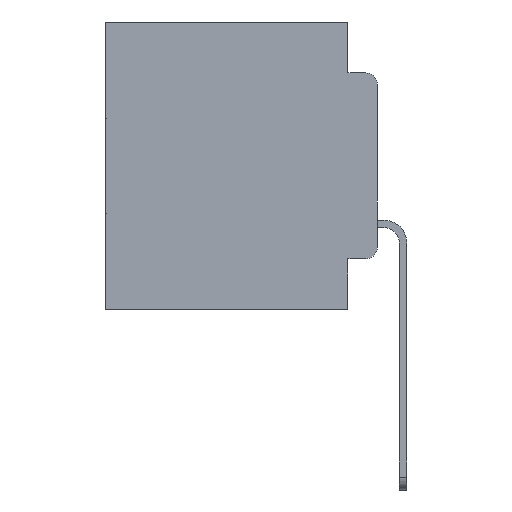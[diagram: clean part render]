
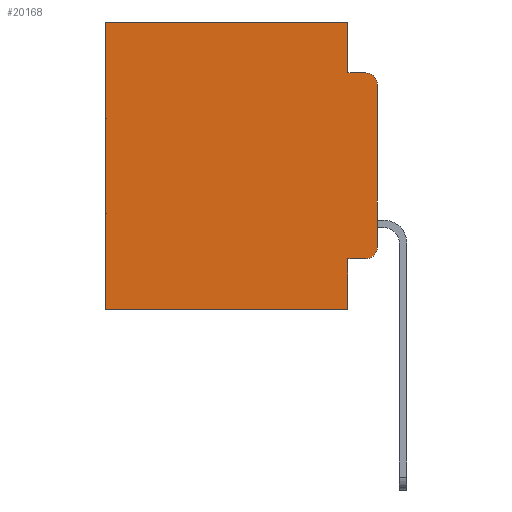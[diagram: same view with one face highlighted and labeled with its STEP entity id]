
A CAD part, left-side view. The second image highlights one B-rep face of the part: STEP entity #20168.
In plain terms, the highlighted planar face has unit normal (-1, 0, 0).
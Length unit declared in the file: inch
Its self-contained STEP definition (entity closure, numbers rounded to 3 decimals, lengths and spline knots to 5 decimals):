
#295 = AXIS2_PLACEMENT_3D ( 'NONE', #25992, #11797, #28371 ) ;
#780 = CARTESIAN_POINT ( 'NONE',  ( 0.298, 0.02, -0.1085 ) ) ;
#937 = DIRECTION ( 'NONE',  ( 0., 0., -1. ) ) ;
#1480 = AXIS2_PLACEMENT_3D ( 'NONE', #780, #18146, #3395 ) ;
#1501 = PLANE ( 'NONE',  #26818 ) ;
#1681 = CARTESIAN_POINT ( 'NONE',  ( 0.298, 0.051, -0.4115 ) ) ;
#2046 = LINE ( 'NONE', #12468, #8830 ) ;
#2179 = CARTESIAN_POINT ( 'NONE',  ( 0.298, 0., 0. ) ) ;
#3289 = ORIENTED_EDGE ( 'NONE', *, *, #7076, .T. ) ;
#3395 = DIRECTION ( 'NONE',  ( 0., 0., -1. ) ) ;
#4110 = DIRECTION ( 'NONE',  ( 0., 0., -1. ) ) ;
#4429 = VECTOR ( 'NONE', #15636, 39.37008 ) ;
#4749 = DIRECTION ( 'NONE',  ( 0., 0., -1. ) ) ;
#4817 = CIRCLE ( 'NONE', #1480, 0.02 ) ;
#5006 = ORIENTED_EDGE ( 'NONE', *, *, #15194, .F. ) ;
#5212 = LINE ( 'NONE', #24694, #30025 ) ;
#6494 = EDGE_CURVE ( 'NONE', #29346, #20848, #4817, .T. ) ;
#7076 = EDGE_CURVE ( 'NONE', #20900, #27724, #20448, .T. ) ;
#8329 = DIRECTION ( 'NONE',  ( 0., -1., 0. ) ) ;
#8442 = ORIENTED_EDGE ( 'NONE', *, *, #24426, .F. ) ;
#8830 = VECTOR ( 'NONE', #28987, 39.37008 ) ;
#9593 = LINE ( 'NONE', #20651, #16039 ) ;
#10194 = EDGE_CURVE ( 'NONE', #16567, #20796, #26242, .T. ) ;
#10408 = ORIENTED_EDGE ( 'NONE', *, *, #10194, .F. ) ;
#10576 = CARTESIAN_POINT ( 'NONE',  ( 0.298, 0., -0.3915 ) ) ;
#11154 = LINE ( 'NONE', #13231, #4429 ) ;
#11532 = CARTESIAN_POINT ( 'NONE',  ( 0.298, 0., 0. ) ) ;
#11797 = DIRECTION ( 'NONE',  ( -1., 0., 0. ) ) ;
#12468 = CARTESIAN_POINT ( 'NONE',  ( 0.298, 0.051, -0.0885 ) ) ;
#12480 = EDGE_CURVE ( 'NONE', #28825, #22556, #21371, .T. ) ;
#12609 = FACE_OUTER_BOUND ( 'NONE', #29238, .T. ) ;
#12735 = VERTEX_POINT ( 'NONE', #10576 ) ;
#12907 = DIRECTION ( 'NONE',  ( 0., 0., -1. ) ) ;
#13231 = CARTESIAN_POINT ( 'NONE',  ( 0.298, 0.051, 0. ) ) ;
#13322 = CIRCLE ( 'NONE', #295, 0.02 ) ;
#13988 = CARTESIAN_POINT ( 'NONE',  ( 0.298, 0.02, -0.0885 ) ) ;
#14141 = VECTOR ( 'NONE', #8329, 39.37008 ) ;
#14692 = EDGE_CURVE ( 'NONE', #22556, #20796, #5212, .T. ) ;
#15078 = VECTOR ( 'NONE', #21134, 39.37008 ) ;
#15194 = EDGE_CURVE ( 'NONE', #29346, #12735, #29265, .T. ) ;
#15424 = CARTESIAN_POINT ( 'NONE',  ( 0.298, 0.473, 0. ) ) ;
#15434 = EDGE_CURVE ( 'NONE', #28825, #20985, #9593, .T. ) ;
#15636 = DIRECTION ( 'NONE',  ( 0., 0., -1. ) ) ;
#16039 = VECTOR ( 'NONE', #937, 39.37008 ) ;
#16567 = VERTEX_POINT ( 'NONE', #26056 ) ;
#18146 = DIRECTION ( 'NONE',  ( -1., 0., 0. ) ) ;
#18563 = CARTESIAN_POINT ( 'NONE',  ( 0.298, 0.473, -0.5 ) ) ;
#18811 = DIRECTION ( 'NONE',  ( 1., 0., 0. ) ) ;
#19173 = CARTESIAN_POINT ( 'NONE',  ( 0.298, 0.051, -0.0885 ) ) ;
#19331 = DIRECTION ( 'NONE',  ( 0., 1., 0. ) ) ;
#20168 = ADVANCED_FACE ( 'NONE', ( #12609 ), #1501, .F. ) ;
#20448 = LINE ( 'NONE', #29713, #14141 ) ;
#20651 = CARTESIAN_POINT ( 'NONE',  ( 0.298, 0.051, 0. ) ) ;
#20796 = VERTEX_POINT ( 'NONE', #18563 ) ;
#20848 = VERTEX_POINT ( 'NONE', #13988 ) ;
#20900 = VERTEX_POINT ( 'NONE', #1681 ) ;
#20939 = CARTESIAN_POINT ( 'NONE',  ( 0.298, 0., -0.1085 ) ) ;
#20985 = VERTEX_POINT ( 'NONE', #19173 ) ;
#21134 = DIRECTION ( 'NONE',  ( 0., 1., 0. ) ) ;
#21371 = LINE ( 'NONE', #11532, #15078 ) ;
#21385 = CARTESIAN_POINT ( 'NONE',  ( 0.298, 0.051, 0. ) ) ;
#21619 = ORIENTED_EDGE ( 'NONE', *, *, #14692, .T. ) ;
#21761 = ORIENTED_EDGE ( 'NONE', *, *, #27824, .F. ) ;
#22556 = VERTEX_POINT ( 'NONE', #15424 ) ;
#22685 = ORIENTED_EDGE ( 'NONE', *, *, #15434, .F. ) ;
#23003 = VECTOR ( 'NONE', #4749, 39.37008 ) ;
#24426 = EDGE_CURVE ( 'NONE', #20900, #16567, #11154, .T. ) ;
#24694 = CARTESIAN_POINT ( 'NONE',  ( 0.298, 0.473, 0. ) ) ;
#25513 = VECTOR ( 'NONE', #19331, 39.37008 ) ;
#25790 = CARTESIAN_POINT ( 'NONE',  ( 0.298, 0., 0. ) ) ;
#25992 = CARTESIAN_POINT ( 'NONE',  ( 0.298, 0.02, -0.3915 ) ) ;
#26056 = CARTESIAN_POINT ( 'NONE',  ( 0.298, 0.051, -0.5 ) ) ;
#26242 = LINE ( 'NONE', #28691, #25513 ) ;
#26531 = ORIENTED_EDGE ( 'NONE', *, *, #6494, .T. ) ;
#26818 = AXIS2_PLACEMENT_3D ( 'NONE', #25790, #18811, #4110 ) ;
#27724 = VERTEX_POINT ( 'NONE', #30935 ) ;
#27824 = EDGE_CURVE ( 'NONE', #20985, #20848, #2046, .T. ) ;
#28371 = DIRECTION ( 'NONE',  ( 0., 0., -1. ) ) ;
#28627 = ORIENTED_EDGE ( 'NONE', *, *, #28788, .T. ) ;
#28691 = CARTESIAN_POINT ( 'NONE',  ( 0.298, 0., -0.5 ) ) ;
#28788 = EDGE_CURVE ( 'NONE', #27724, #12735, #13322, .T. ) ;
#28825 = VERTEX_POINT ( 'NONE', #21385 ) ;
#28987 = DIRECTION ( 'NONE',  ( 0., -1., 0. ) ) ;
#29238 = EDGE_LOOP ( 'NONE', ( #5006, #26531, #21761, #22685, #29685, #21619, #10408, #8442, #3289, #28627 ) ) ;
#29265 = LINE ( 'NONE', #2179, #23003 ) ;
#29346 = VERTEX_POINT ( 'NONE', #20939 ) ;
#29685 = ORIENTED_EDGE ( 'NONE', *, *, #12480, .T. ) ;
#29713 = CARTESIAN_POINT ( 'NONE',  ( 0.298, 0.051, -0.4115 ) ) ;
#30025 = VECTOR ( 'NONE', #12907, 39.37008 ) ;
#30935 = CARTESIAN_POINT ( 'NONE',  ( 0.298, 0.02, -0.4115 ) ) ;
